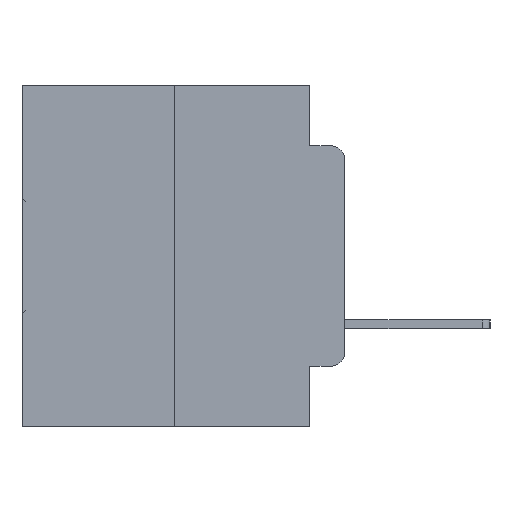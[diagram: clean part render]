
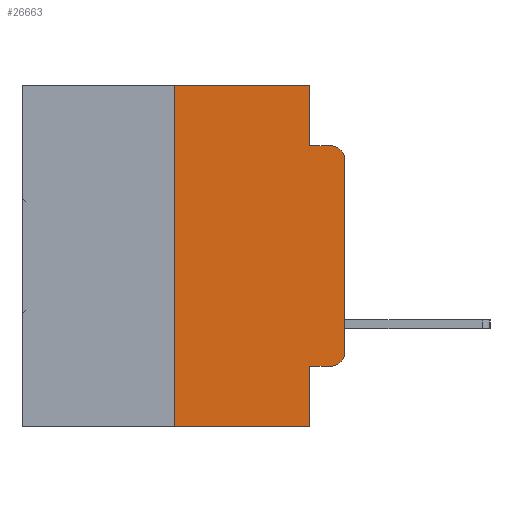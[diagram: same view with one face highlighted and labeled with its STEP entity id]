
A CAD part, left-side view. The second image highlights one B-rep face of the part: STEP entity #26663.
In plain terms, the highlighted planar face has unit normal (-1, 0, 0).
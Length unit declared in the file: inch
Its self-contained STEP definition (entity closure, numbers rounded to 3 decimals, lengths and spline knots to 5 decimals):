
#29 = DIRECTION ( 'NONE',  ( 0., 0., -1. ) ) ;
#246 = EDGE_CURVE ( 'NONE', #14677, #5074, #16525, .T. ) ;
#334 = DIRECTION ( 'NONE',  ( 0., -1., 0. ) ) ;
#383 = EDGE_CURVE ( 'NONE', #27265, #5074, #28980, .T. ) ;
#732 = CARTESIAN_POINT ( 'NONE',  ( 0., 0.051, -0.4115 ) ) ;
#795 = ORIENTED_EDGE ( 'NONE', *, *, #11852, .T. ) ;
#950 = AXIS2_PLACEMENT_3D ( 'NONE', #20165, #3175, #23100 ) ;
#1154 = VERTEX_POINT ( 'NONE', #21276 ) ;
#1270 = ORIENTED_EDGE ( 'NONE', *, *, #246, .F. ) ;
#1474 = CARTESIAN_POINT ( 'NONE',  ( 0., 0.051, 0. ) ) ;
#1584 = DIRECTION ( 'NONE',  ( 0., 0., 1. ) ) ;
#1836 = FACE_OUTER_BOUND ( 'NONE', #6449, .T. ) ;
#3175 = DIRECTION ( 'NONE',  ( -1., 0., 0. ) ) ;
#3371 = VERTEX_POINT ( 'NONE', #13889 ) ;
#3524 = ORIENTED_EDGE ( 'NONE', *, *, #15709, .T. ) ;
#3831 = ORIENTED_EDGE ( 'NONE', *, *, #14760, .F. ) ;
#4398 = CARTESIAN_POINT ( 'NONE',  ( 0., 0., -0.1085 ) ) ;
#5074 = VERTEX_POINT ( 'NONE', #27005 ) ;
#5251 = AXIS2_PLACEMENT_3D ( 'NONE', #6756, #23186, #9211 ) ;
#5388 = DIRECTION ( 'NONE',  ( 0., -1., 0. ) ) ;
#5529 = LINE ( 'NONE', #26351, #19621 ) ;
#5602 = DIRECTION ( 'NONE',  ( 0., -1., 0. ) ) ;
#5862 = VECTOR ( 'NONE', #1584, 39.37008 ) ;
#6389 = LINE ( 'NONE', #26393, #24338 ) ;
#6449 = EDGE_LOOP ( 'NONE', ( #795, #7686, #1270, #7595, #18337, #3831, #3524, #13443, #24134, #21965 ) ) ;
#6756 = CARTESIAN_POINT ( 'NONE',  ( 0., 0.02, -0.3915 ) ) ;
#7595 = ORIENTED_EDGE ( 'NONE', *, *, #17997, .F. ) ;
#7686 = ORIENTED_EDGE ( 'NONE', *, *, #383, .T. ) ;
#7740 = DIRECTION ( 'NONE',  ( 0., 0., -1. ) ) ;
#8822 = VERTEX_POINT ( 'NONE', #19796 ) ;
#9119 = VERTEX_POINT ( 'NONE', #11450 ) ;
#9211 = DIRECTION ( 'NONE',  ( 0., 0., -1. ) ) ;
#9553 = VECTOR ( 'NONE', #27838, 39.37008 ) ;
#9865 = VERTEX_POINT ( 'NONE', #14169 ) ;
#10042 = EDGE_CURVE ( 'NONE', #3371, #9865, #6389, .T. ) ;
#11450 = CARTESIAN_POINT ( 'NONE',  ( 0., 0.25, -0.5 ) ) ;
#11852 = EDGE_CURVE ( 'NONE', #8822, #27265, #24962, .T. ) ;
#11862 = EDGE_CURVE ( 'NONE', #27520, #13779, #5529, .T. ) ;
#11885 = VECTOR ( 'NONE', #12485, 39.37008 ) ;
#12220 = LINE ( 'NONE', #29524, #5862 ) ;
#12324 = CARTESIAN_POINT ( 'NONE',  ( 0., 0.473, -0.5 ) ) ;
#12485 = DIRECTION ( 'NONE',  ( 0., 0., 1. ) ) ;
#12579 = CARTESIAN_POINT ( 'NONE',  ( 0., 0.25, 0. ) ) ;
#13443 = ORIENTED_EDGE ( 'NONE', *, *, #10042, .F. ) ;
#13779 = VERTEX_POINT ( 'NONE', #26826 ) ;
#13889 = CARTESIAN_POINT ( 'NONE',  ( 0., 0.051, -0.4115 ) ) ;
#14169 = CARTESIAN_POINT ( 'NONE',  ( 0., 0.051, -0.5 ) ) ;
#14240 = CARTESIAN_POINT ( 'NONE',  ( 0., 0.051, -0.0885 ) ) ;
#14257 = VECTOR ( 'NONE', #5602, 39.37008 ) ;
#14391 = DIRECTION ( 'NONE',  ( 1., 0., 0. ) ) ;
#14677 = VERTEX_POINT ( 'NONE', #24752 ) ;
#14760 = EDGE_CURVE ( 'NONE', #9119, #27520, #12220, .T. ) ;
#15319 = VECTOR ( 'NONE', #18155, 39.37008 ) ;
#15709 = EDGE_CURVE ( 'NONE', #9119, #9865, #22380, .T. ) ;
#16525 = LINE ( 'NONE', #14240, #9553 ) ;
#16660 = CARTESIAN_POINT ( 'NONE',  ( 0., 0.473, 0. ) ) ;
#17997 = EDGE_CURVE ( 'NONE', #13779, #14677, #20836, .T. ) ;
#18155 = DIRECTION ( 'NONE',  ( 0., 0., -1. ) ) ;
#18181 = CIRCLE ( 'NONE', #5251, 0.02 ) ;
#18337 = ORIENTED_EDGE ( 'NONE', *, *, #11862, .F. ) ;
#19621 = VECTOR ( 'NONE', #5388, 39.37008 ) ;
#19796 = CARTESIAN_POINT ( 'NONE',  ( 0., 0., -0.3915 ) ) ;
#20165 = CARTESIAN_POINT ( 'NONE',  ( 0., 0.02, -0.1085 ) ) ;
#20836 = LINE ( 'NONE', #1474, #15319 ) ;
#21276 = CARTESIAN_POINT ( 'NONE',  ( 0., 0.02, -0.4115 ) ) ;
#21965 = ORIENTED_EDGE ( 'NONE', *, *, #22522, .T. ) ;
#22380 = LINE ( 'NONE', #12324, #27677 ) ;
#22522 = EDGE_CURVE ( 'NONE', #1154, #8822, #18181, .T. ) ;
#23035 = AXIS2_PLACEMENT_3D ( 'NONE', #16660, #14391, #29 ) ;
#23100 = DIRECTION ( 'NONE',  ( 0., 0., -1. ) ) ;
#23186 = DIRECTION ( 'NONE',  ( -1., 0., 0. ) ) ;
#23629 = PLANE ( 'NONE',  #23035 ) ;
#24043 = CARTESIAN_POINT ( 'NONE',  ( 0., 0., 0. ) ) ;
#24134 = ORIENTED_EDGE ( 'NONE', *, *, #25578, .T. ) ;
#24338 = VECTOR ( 'NONE', #7740, 39.37008 ) ;
#24752 = CARTESIAN_POINT ( 'NONE',  ( 0., 0.051, -0.0885 ) ) ;
#24962 = LINE ( 'NONE', #24043, #11885 ) ;
#25578 = EDGE_CURVE ( 'NONE', #3371, #1154, #26547, .T. ) ;
#26351 = CARTESIAN_POINT ( 'NONE',  ( 0., 0.473, 0. ) ) ;
#26393 = CARTESIAN_POINT ( 'NONE',  ( 0., 0.051, 0. ) ) ;
#26547 = LINE ( 'NONE', #732, #14257 ) ;
#26663 = ADVANCED_FACE ( 'NONE', ( #1836 ), #23629, .F. ) ;
#26826 = CARTESIAN_POINT ( 'NONE',  ( 0., 0.051, 0. ) ) ;
#27005 = CARTESIAN_POINT ( 'NONE',  ( 0., 0.02, -0.0885 ) ) ;
#27265 = VERTEX_POINT ( 'NONE', #4398 ) ;
#27520 = VERTEX_POINT ( 'NONE', #12579 ) ;
#27677 = VECTOR ( 'NONE', #334, 39.37008 ) ;
#27838 = DIRECTION ( 'NONE',  ( 0., -1., 0. ) ) ;
#28980 = CIRCLE ( 'NONE', #950, 0.02 ) ;
#29524 = CARTESIAN_POINT ( 'NONE',  ( 0., 0.25, 0. ) ) ;
